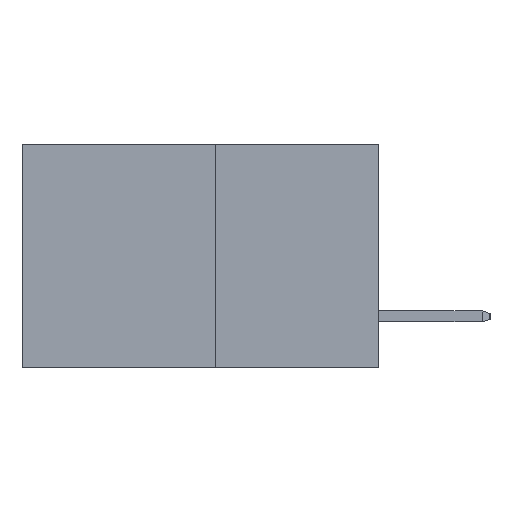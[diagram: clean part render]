
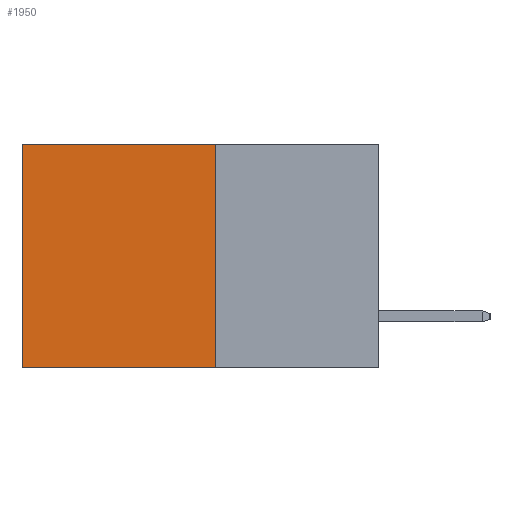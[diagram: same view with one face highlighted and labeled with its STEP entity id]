
A CAD part, left-side view. The second image highlights one B-rep face of the part: STEP entity #1950.
In plain terms, the highlighted planar face has unit normal (-1, 0, 0).
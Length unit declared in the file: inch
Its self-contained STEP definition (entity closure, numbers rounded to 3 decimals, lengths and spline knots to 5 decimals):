
#515 = FACE_OUTER_BOUND ( 'NONE', #4655, .T. ) ;
#819 = ORIENTED_EDGE ( 'NONE', *, *, #8438, .F. ) ;
#963 = CARTESIAN_POINT ( 'NONE',  ( 0.277, 0.59, -0.37 ) ) ;
#1023 = DIRECTION ( 'NONE',  ( 0., 0., -1. ) ) ;
#1197 = LINE ( 'NONE', #13796, #6301 ) ;
#1273 = LINE ( 'NONE', #10591, #6684 ) ;
#1409 = LINE ( 'NONE', #12559, #12469 ) ;
#1950 = ADVANCED_FACE ( 'NONE', ( #515 ), #9187, .F. ) ;
#2314 = CARTESIAN_POINT ( 'NONE',  ( 0.277, 0.27, -0.37 ) ) ;
#2606 = CARTESIAN_POINT ( 'NONE',  ( 0.277, 0.27, 0. ) ) ;
#3240 = VERTEX_POINT ( 'NONE', #2314 ) ;
#4485 = CARTESIAN_POINT ( 'NONE',  ( 0.277, 0.59, 0. ) ) ;
#4655 = EDGE_LOOP ( 'NONE', ( #7154, #819, #7031, #5046 ) ) ;
#5046 = ORIENTED_EDGE ( 'NONE', *, *, #13313, .T. ) ;
#5385 = VECTOR ( 'NONE', #10109, 39.37008 ) ;
#5890 = VERTEX_POINT ( 'NONE', #13628 ) ;
#6301 = VECTOR ( 'NONE', #1023, 39.37008 ) ;
#6684 = VECTOR ( 'NONE', #11652, 39.37008 ) ;
#7031 = ORIENTED_EDGE ( 'NONE', *, *, #9431, .F. ) ;
#7154 = ORIENTED_EDGE ( 'NONE', *, *, #13605, .T. ) ;
#8026 = VERTEX_POINT ( 'NONE', #4485 ) ;
#8438 = EDGE_CURVE ( 'NONE', #3240, #11823, #1409, .T. ) ;
#8965 = DIRECTION ( 'NONE',  ( 0., 0., -1. ) ) ;
#9071 = DIRECTION ( 'NONE',  ( 1., 0., 0. ) ) ;
#9187 = PLANE ( 'NONE',  #13701 ) ;
#9431 = EDGE_CURVE ( 'NONE', #5890, #3240, #1197, .T. ) ;
#9768 = CARTESIAN_POINT ( 'NONE',  ( 0.277, 0.27, -0.37 ) ) ;
#10109 = DIRECTION ( 'NONE',  ( 0., 1., 0. ) ) ;
#10591 = CARTESIAN_POINT ( 'NONE',  ( 0.277, 0.59, -0.37 ) ) ;
#10705 = LINE ( 'NONE', #2606, #5385 ) ;
#11652 = DIRECTION ( 'NONE',  ( 0., 0., -1. ) ) ;
#11823 = VERTEX_POINT ( 'NONE', #963 ) ;
#12469 = VECTOR ( 'NONE', #13578, 39.37008 ) ;
#12559 = CARTESIAN_POINT ( 'NONE',  ( 0.277, 0.27, -0.37 ) ) ;
#13313 = EDGE_CURVE ( 'NONE', #5890, #8026, #10705, .T. ) ;
#13578 = DIRECTION ( 'NONE',  ( 0., 1., 0. ) ) ;
#13605 = EDGE_CURVE ( 'NONE', #8026, #11823, #1273, .T. ) ;
#13628 = CARTESIAN_POINT ( 'NONE',  ( 0.277, 0.27, 0. ) ) ;
#13701 = AXIS2_PLACEMENT_3D ( 'NONE', #9768, #9071, #8965 ) ;
#13796 = CARTESIAN_POINT ( 'NONE',  ( 0.277, 0.27, -0.37 ) ) ;
